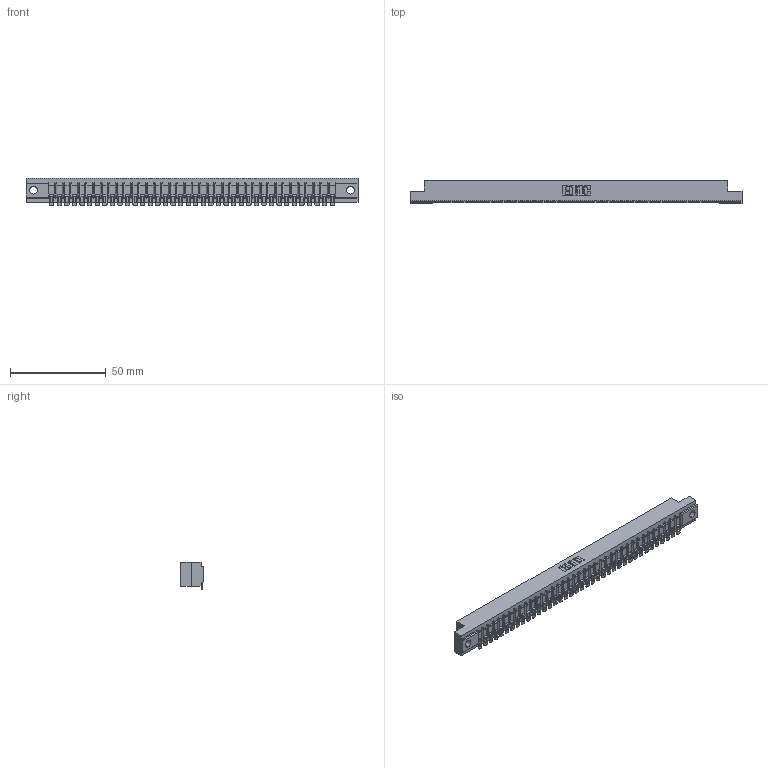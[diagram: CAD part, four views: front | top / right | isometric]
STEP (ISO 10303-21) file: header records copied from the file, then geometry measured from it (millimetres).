
FILE_DESCRIPTION (( 'STEP AP203' ), '1' );
FILE_NAME ('357-038-554-104.STEP', '2019-09-17T07:59:53', ( '' ), ( '' ), 'SwSTEP 2.0', 'SolidWorks 2016', '' );
FILE_SCHEMA (( 'CONFIG_CONTROL_DESIGN' ));
Length unit declared in the file: inch
Products named in the file (3): 357-038-554-104; 307 Part_.156 Dia Mounting Holes; 307-290-002_554
Assembly tree (39 placements, depth 2):
  357-038-554-104
    307 Part_.156 Dia Mounting Holes
    307-290-002_554  x38
Bounding box: 173.58 x 12.01 x 14.52 mm (x, y, z)
Volume: 18453.6 mm3; surface area: 23097.3 mm2
Topology: 39 solids, 39 shells, 3249 faces, 9973 edges, 6542 vertices
Faces by surface type: plane 1832, cylinder 1339, sphere 78
Entity records: 34453 total; most frequent: CARTESIAN_POINT 5816, ORIENTED_EDGE 5804, DIRECTION 5650, EDGE_CURVE 2902, LINE 2222, VECTOR 2222, VERTEX_POINT 1880, AXIS2_PLACEMENT_3D 1714
